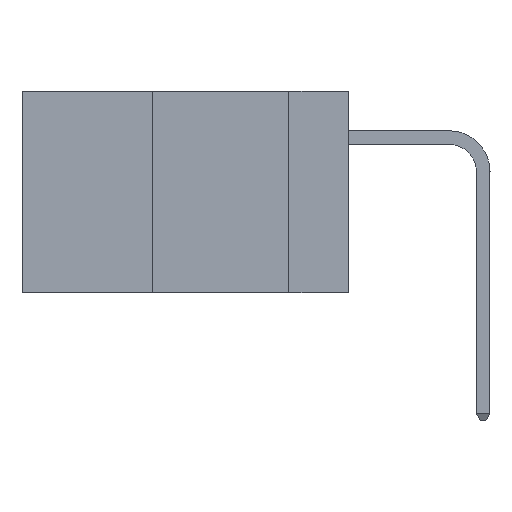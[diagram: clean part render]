
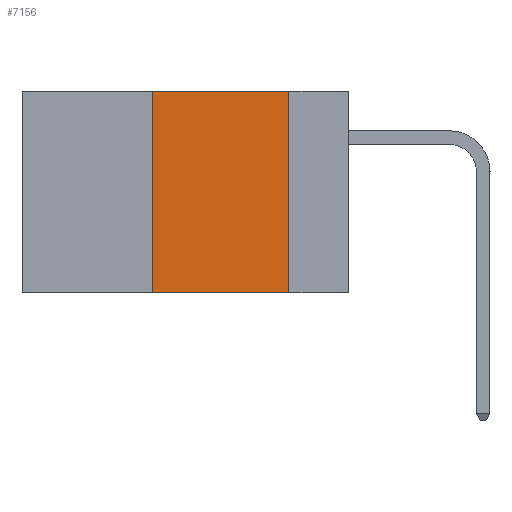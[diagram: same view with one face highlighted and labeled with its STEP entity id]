
A CAD part, left-side view. The second image highlights one B-rep face of the part: STEP entity #7156.
In plain terms, the highlighted planar face has unit normal (-1, 0, 0).
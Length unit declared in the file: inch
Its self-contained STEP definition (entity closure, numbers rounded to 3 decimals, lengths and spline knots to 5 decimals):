
#148 = VERTEX_POINT ( 'NONE', #5747 ) ;
#254 = LINE ( 'NONE', #3645, #7588 ) ;
#652 = VERTEX_POINT ( 'NONE', #3406 ) ;
#978 = PLANE ( 'NONE',  #4323 ) ;
#1028 = LINE ( 'NONE', #2840, #7892 ) ;
#1187 = CARTESIAN_POINT ( 'NONE',  ( 0., 0.36, 0. ) ) ;
#2106 = VECTOR ( 'NONE', #7507, 39.37008 ) ;
#2548 = EDGE_CURVE ( 'NONE', #652, #7948, #1028, .T. ) ;
#2574 = LINE ( 'NONE', #6758, #2106 ) ;
#2795 = EDGE_CURVE ( 'NONE', #148, #7948, #3071, .T. ) ;
#2840 = CARTESIAN_POINT ( 'NONE',  ( 0., 0.11, 0. ) ) ;
#2901 = DIRECTION ( 'NONE',  ( 0., -1., 0. ) ) ;
#3071 = LINE ( 'NONE', #8052, #8726 ) ;
#3280 = VERTEX_POINT ( 'NONE', #1187 ) ;
#3406 = CARTESIAN_POINT ( 'NONE',  ( 0., 0.11, 0. ) ) ;
#3616 = FACE_OUTER_BOUND ( 'NONE', #5979, .T. ) ;
#3645 = CARTESIAN_POINT ( 'NONE',  ( 0., 0.36, 0. ) ) ;
#4323 = AXIS2_PLACEMENT_3D ( 'NONE', #9164, #4749, #4786 ) ;
#4685 = EDGE_CURVE ( 'NONE', #148, #3280, #254, .T. ) ;
#4749 = DIRECTION ( 'NONE',  ( 1., 0., 0. ) ) ;
#4786 = DIRECTION ( 'NONE',  ( 0., 0., -1. ) ) ;
#5283 = ORIENTED_EDGE ( 'NONE', *, *, #2548, .F. ) ;
#5729 = DIRECTION ( 'NONE',  ( 0., 0., -1. ) ) ;
#5747 = CARTESIAN_POINT ( 'NONE',  ( 0., 0.36, -0.37 ) ) ;
#5874 = EDGE_CURVE ( 'NONE', #3280, #652, #2574, .T. ) ;
#5979 = EDGE_LOOP ( 'NONE', ( #5283, #6097, #9383, #7360 ) ) ;
#6097 = ORIENTED_EDGE ( 'NONE', *, *, #5874, .F. ) ;
#6758 = CARTESIAN_POINT ( 'NONE',  ( 0., 0.6, 0. ) ) ;
#7156 = ADVANCED_FACE ( 'NONE', ( #3616 ), #978, .F. ) ;
#7360 = ORIENTED_EDGE ( 'NONE', *, *, #2795, .T. ) ;
#7507 = DIRECTION ( 'NONE',  ( 0., -1., 0. ) ) ;
#7588 = VECTOR ( 'NONE', #8146, 39.37008 ) ;
#7683 = CARTESIAN_POINT ( 'NONE',  ( 0., 0.11, -0.37 ) ) ;
#7892 = VECTOR ( 'NONE', #5729, 39.37008 ) ;
#7948 = VERTEX_POINT ( 'NONE', #7683 ) ;
#8052 = CARTESIAN_POINT ( 'NONE',  ( 0., 0.6, -0.37 ) ) ;
#8146 = DIRECTION ( 'NONE',  ( 0., 0., 1. ) ) ;
#8726 = VECTOR ( 'NONE', #2901, 39.37008 ) ;
#9164 = CARTESIAN_POINT ( 'NONE',  ( 0., 0.6, 0. ) ) ;
#9383 = ORIENTED_EDGE ( 'NONE', *, *, #4685, .F. ) ;
